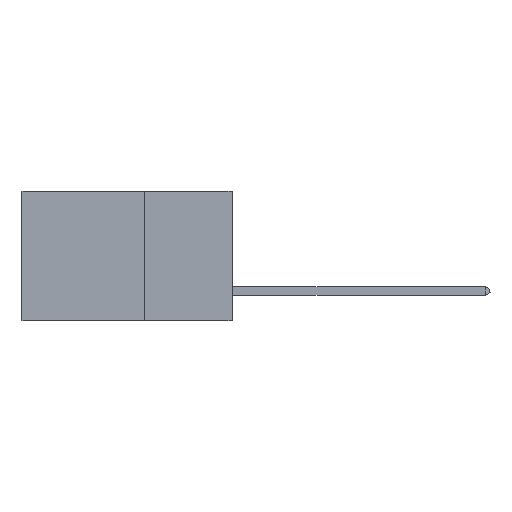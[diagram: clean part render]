
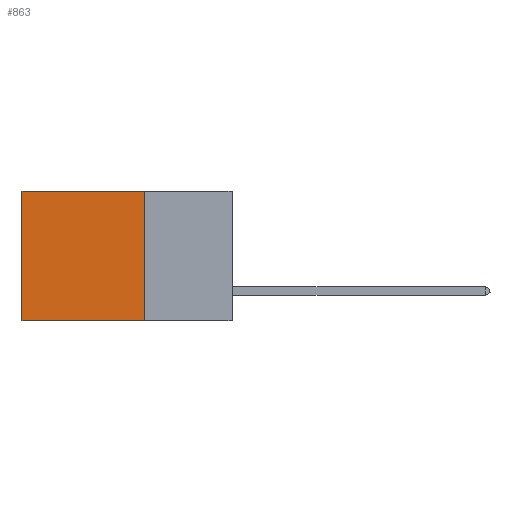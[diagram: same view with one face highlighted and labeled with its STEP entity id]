
A CAD part, left-side view. The second image highlights one B-rep face of the part: STEP entity #863.
In plain terms, the highlighted planar face has unit normal (-1, 0, 0).
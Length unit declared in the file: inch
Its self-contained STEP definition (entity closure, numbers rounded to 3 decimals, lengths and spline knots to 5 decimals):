
#863 = ADVANCED_FACE ( 'NONE', ( #11334 ), #20178, .F. ) ;
#1178 = LINE ( 'NONE', #9411, #23537 ) ;
#1509 = VECTOR ( 'NONE', #23733, 39.37008 ) ;
#2416 = VERTEX_POINT ( 'NONE', #16885 ) ;
#3014 = EDGE_CURVE ( 'NONE', #2416, #13567, #15906, .T. ) ;
#3068 = DIRECTION ( 'NONE',  ( 0., 1., 0. ) ) ;
#3311 = AXIS2_PLACEMENT_3D ( 'NONE', #7331, #22702, #18341 ) ;
#7331 = CARTESIAN_POINT ( 'NONE',  ( 0.2875, 0.25, 0. ) ) ;
#7989 = DIRECTION ( 'NONE',  ( 0., 1., 0. ) ) ;
#8086 = CARTESIAN_POINT ( 'NONE',  ( 0.2875, 0.25, 0. ) ) ;
#9243 = ORIENTED_EDGE ( 'NONE', *, *, #10333, .T. ) ;
#9411 = CARTESIAN_POINT ( 'NONE',  ( 0.2875, 0.25, -0.37 ) ) ;
#10333 = EDGE_CURVE ( 'NONE', #22210, #2416, #17288, .T. ) ;
#11334 = FACE_OUTER_BOUND ( 'NONE', #24649, .T. ) ;
#12995 = ORIENTED_EDGE ( 'NONE', *, *, #23429, .F. ) ;
#13567 = VERTEX_POINT ( 'NONE', #24478 ) ;
#15183 = LINE ( 'NONE', #25001, #22791 ) ;
#15232 = VECTOR ( 'NONE', #7989, 39.37008 ) ;
#15906 = LINE ( 'NONE', #23924, #1509 ) ;
#16353 = DIRECTION ( 'NONE',  ( 0., 0., -1. ) ) ;
#16885 = CARTESIAN_POINT ( 'NONE',  ( 0.2875, 0.6, 0. ) ) ;
#17288 = LINE ( 'NONE', #8086, #15232 ) ;
#18341 = DIRECTION ( 'NONE',  ( 0., 0., -1. ) ) ;
#20178 = PLANE ( 'NONE',  #3311 ) ;
#21498 = CARTESIAN_POINT ( 'NONE',  ( 0.2875, 0.25, 0. ) ) ;
#22210 = VERTEX_POINT ( 'NONE', #21498 ) ;
#22702 = DIRECTION ( 'NONE',  ( 1., 0., 0. ) ) ;
#22791 = VECTOR ( 'NONE', #16353, 39.37008 ) ;
#23429 = EDGE_CURVE ( 'NONE', #22210, #25149, #15183, .T. ) ;
#23537 = VECTOR ( 'NONE', #3068, 39.37008 ) ;
#23733 = DIRECTION ( 'NONE',  ( 0., 0., -1. ) ) ;
#23924 = CARTESIAN_POINT ( 'NONE',  ( 0.2875, 0.6, 0. ) ) ;
#24478 = CARTESIAN_POINT ( 'NONE',  ( 0.2875, 0.6, -0.37 ) ) ;
#24649 = EDGE_LOOP ( 'NONE', ( #27805, #27258, #12995, #9243 ) ) ;
#25001 = CARTESIAN_POINT ( 'NONE',  ( 0.2875, 0.25, 0. ) ) ;
#25149 = VERTEX_POINT ( 'NONE', #27712 ) ;
#25771 = EDGE_CURVE ( 'NONE', #25149, #13567, #1178, .T. ) ;
#27258 = ORIENTED_EDGE ( 'NONE', *, *, #25771, .F. ) ;
#27712 = CARTESIAN_POINT ( 'NONE',  ( 0.2875, 0.25, -0.37 ) ) ;
#27805 = ORIENTED_EDGE ( 'NONE', *, *, #3014, .T. ) ;
